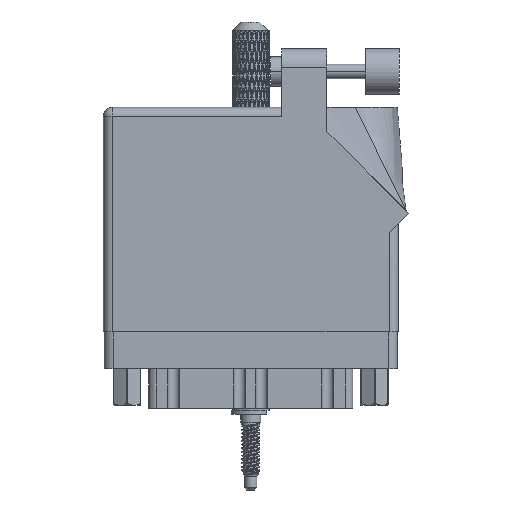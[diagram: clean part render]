
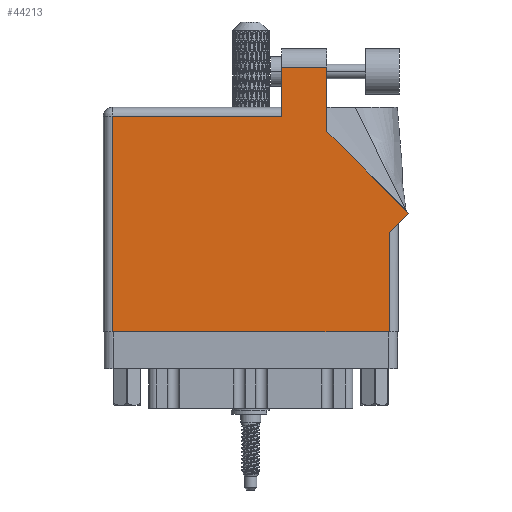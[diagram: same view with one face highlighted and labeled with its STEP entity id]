
A CAD part, front view. The second image highlights one B-rep face of the part: STEP entity #44213.
In plain terms, the highlighted face is planar.
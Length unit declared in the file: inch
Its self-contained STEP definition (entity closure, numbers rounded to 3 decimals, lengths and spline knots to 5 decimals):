
#605 = EDGE_LOOP ( 'NONE', ( #22197, #103192, #86689, #50129, #4848, #37556, #25221, #12216, #58622 ) ) ;
#909 = EDGE_CURVE ( 'NONE', #11735, #4283, #110877, .T. ) ;
#1513 = DIRECTION ( 'NONE',  ( -0.707, 0.707, 0. ) ) ;
#3032 = CARTESIAN_POINT ( 'NONE',  ( 0.062, 0., 0. ) ) ;
#4283 = VERTEX_POINT ( 'NONE', #112407 ) ;
#4608 = LINE ( 'NONE', #39561, #52473 ) ;
#4848 = ORIENTED_EDGE ( 'NONE', *, *, #24485, .T. ) ;
#5038 = CARTESIAN_POINT ( 'NONE',  ( 1.217, 1.468, 0. ) ) ;
#6625 = CARTESIAN_POINT ( 'NONE',  ( 2.01, 0.737, 0. ) ) ;
#9337 = AXIS2_PLACEMENT_3D ( 'NONE', #59095, #94024, #68254 ) ;
#10555 = EDGE_CURVE ( 'NONE', #108343, #88633, #45053, .T. ) ;
#11735 = VERTEX_POINT ( 'NONE', #100679 ) ;
#12216 = ORIENTED_EDGE ( 'NONE', *, *, #13080, .T. ) ;
#13080 = EDGE_CURVE ( 'NONE', #4283, #108343, #15234, .T. ) ;
#14219 = VECTOR ( 'NONE', #78175, 39.37008 ) ;
#14301 = VERTEX_POINT ( 'NONE', #72094 ) ;
#15234 = LINE ( 'NONE', #6625, #77655 ) ;
#18014 = DIRECTION ( 'NONE',  ( 0., -1., 0. ) ) ;
#19288 = CARTESIAN_POINT ( 'NONE',  ( 2.08071, 0.80771, 0. ) ) ;
#22197 = ORIENTED_EDGE ( 'NONE', *, *, #36648, .T. ) ;
#22732 = DIRECTION ( 'NONE',  ( 0., 1., 0. ) ) ;
#24485 = EDGE_CURVE ( 'NONE', #14301, #75940, #62414, .T. ) ;
#25221 = ORIENTED_EDGE ( 'NONE', *, *, #909, .T. ) ;
#29443 = CARTESIAN_POINT ( 'NONE',  ( 1.217, 1.53, 0. ) ) ;
#36648 = EDGE_CURVE ( 'NONE', #88633, #37971, #51259, .T. ) ;
#37556 = ORIENTED_EDGE ( 'NONE', *, *, #99201, .T. ) ;
#37971 = VERTEX_POINT ( 'NONE', #78207 ) ;
#38528 = VERTEX_POINT ( 'NONE', #64542 ) ;
#39561 = CARTESIAN_POINT ( 'NONE',  ( 0., 0., 0. ) ) ;
#40632 = VECTOR ( 'NONE', #84473, 39.37008 ) ;
#41686 = VECTOR ( 'NONE', #22732, 39.37008 ) ;
#42639 = CARTESIAN_POINT ( 'NONE',  ( 1.524, 1.36442, 0. ) ) ;
#44213 = ADVANCED_FACE ( 'NONE', ( #67686 ), #102612, .F. ) ;
#45053 = LINE ( 'NONE', #19288, #99276 ) ;
#47566 = VERTEX_POINT ( 'NONE', #5038 ) ;
#49516 = LINE ( 'NONE', #50088, #40632 ) ;
#50088 = CARTESIAN_POINT ( 'NONE',  ( 0., 1.468, 0. ) ) ;
#50129 = ORIENTED_EDGE ( 'NONE', *, *, #61158, .T. ) ;
#51259 = LINE ( 'NONE', #103954, #14219 ) ;
#52473 = VECTOR ( 'NONE', #74487, 39.37008 ) ;
#58622 = ORIENTED_EDGE ( 'NONE', *, *, #10555, .T. ) ;
#59095 = CARTESIAN_POINT ( 'NONE',  ( 0., 1.53, 0. ) ) ;
#60673 = VECTOR ( 'NONE', #69412, 39.37008 ) ;
#61158 = EDGE_CURVE ( 'NONE', #47566, #14301, #49516, .T. ) ;
#62414 = LINE ( 'NONE', #62969, #108464 ) ;
#62969 = CARTESIAN_POINT ( 'NONE',  ( 0.062, 0., 0. ) ) ;
#64542 = CARTESIAN_POINT ( 'NONE',  ( 1.217, 1.805, 0. ) ) ;
#66217 = CARTESIAN_POINT ( 'NONE',  ( 1.948, 0.737, 0. ) ) ;
#67686 = FACE_OUTER_BOUND ( 'NONE', #605, .T. ) ;
#68254 = DIRECTION ( 'NONE',  ( -1., 0., 0. ) ) ;
#69412 = DIRECTION ( 'NONE',  ( -1., 0., 0. ) ) ;
#69959 = VECTOR ( 'NONE', #18014, 39.37008 ) ;
#72094 = CARTESIAN_POINT ( 'NONE',  ( 0.062, 1.468, 0. ) ) ;
#74487 = DIRECTION ( 'NONE',  ( 1., 0., 0. ) ) ;
#75940 = VERTEX_POINT ( 'NONE', #3032 ) ;
#77655 = VECTOR ( 'NONE', #103402, 39.37008 ) ;
#78175 = DIRECTION ( 'NONE',  ( 0., 1., 0. ) ) ;
#78207 = CARTESIAN_POINT ( 'NONE',  ( 1.524, 1.805, 0. ) ) ;
#84473 = DIRECTION ( 'NONE',  ( -1., 0., 0. ) ) ;
#86689 = ORIENTED_EDGE ( 'NONE', *, *, #90953, .T. ) ;
#88633 = VERTEX_POINT ( 'NONE', #42639 ) ;
#89071 = EDGE_CURVE ( 'NONE', #37971, #38528, #105479, .T. ) ;
#90953 = EDGE_CURVE ( 'NONE', #38528, #47566, #107858, .T. ) ;
#94024 = DIRECTION ( 'NONE',  ( 0., 0., -1. ) ) ;
#96299 = CARTESIAN_POINT ( 'NONE',  ( 1.217, 1.805, 0. ) ) ;
#96898 = CARTESIAN_POINT ( 'NONE',  ( 2.08071, 0.80771, 0. ) ) ;
#99201 = EDGE_CURVE ( 'NONE', #75940, #11735, #4608, .T. ) ;
#99276 = VECTOR ( 'NONE', #1513, 39.37008 ) ;
#100679 = CARTESIAN_POINT ( 'NONE',  ( 1.948, 0., 0. ) ) ;
#102612 = PLANE ( 'NONE',  #9337 ) ;
#103192 = ORIENTED_EDGE ( 'NONE', *, *, #89071, .T. ) ;
#103402 = DIRECTION ( 'NONE',  ( 0.707, 0.707, 0. ) ) ;
#103954 = CARTESIAN_POINT ( 'NONE',  ( 1.524, 1.36442, 0. ) ) ;
#105479 = LINE ( 'NONE', #96299, #60673 ) ;
#107057 = DIRECTION ( 'NONE',  ( 0., -1., 0. ) ) ;
#107858 = LINE ( 'NONE', #29443, #69959 ) ;
#108343 = VERTEX_POINT ( 'NONE', #96898 ) ;
#108464 = VECTOR ( 'NONE', #107057, 39.37008 ) ;
#110877 = LINE ( 'NONE', #66217, #41686 ) ;
#112407 = CARTESIAN_POINT ( 'NONE',  ( 1.948, 0.675, 0. ) ) ;
